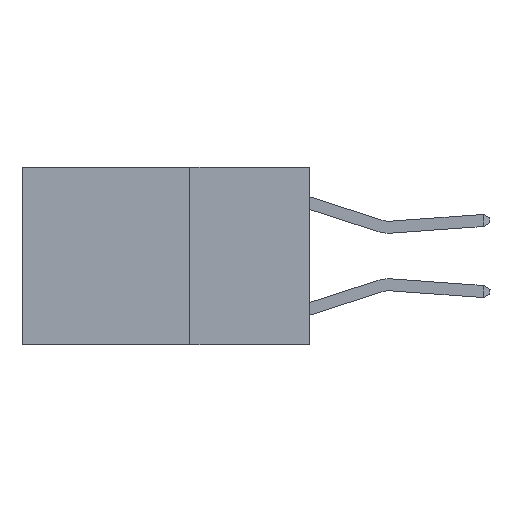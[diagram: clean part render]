
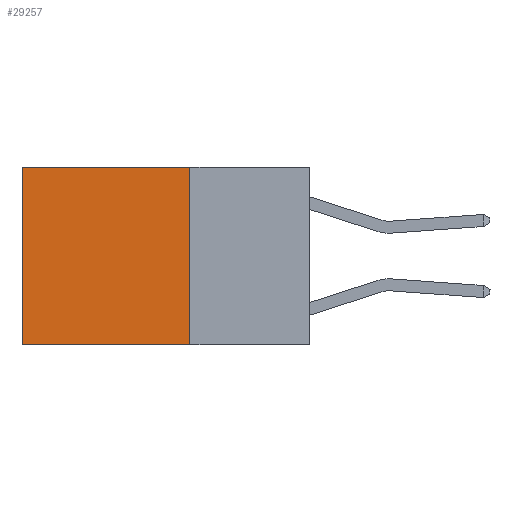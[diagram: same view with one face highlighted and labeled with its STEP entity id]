
A CAD part, left-side view. The second image highlights one B-rep face of the part: STEP entity #29257.
In plain terms, the highlighted planar face has unit normal (-1, 0, 0).
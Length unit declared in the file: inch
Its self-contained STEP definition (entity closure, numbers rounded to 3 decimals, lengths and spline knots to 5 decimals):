
#16 = VERTEX_POINT ( 'NONE', #10404 ) ;
#729 = VECTOR ( 'NONE', #4383, 39.37008 ) ;
#1619 = CARTESIAN_POINT ( 'NONE',  ( 0.2625, 0.25, -0.37 ) ) ;
#1947 = DIRECTION ( 'NONE',  ( 0., 0., -1. ) ) ;
#2571 = AXIS2_PLACEMENT_3D ( 'NONE', #29597, #22573, #27532 ) ;
#2714 = ORIENTED_EDGE ( 'NONE', *, *, #2719, .F. ) ;
#2719 = EDGE_CURVE ( 'NONE', #16, #14542, #9304, .T. ) ;
#4383 = DIRECTION ( 'NONE',  ( 0., 1., 0. ) ) ;
#5448 = FACE_OUTER_BOUND ( 'NONE', #6507, .T. ) ;
#6227 = DIRECTION ( 'NONE',  ( 0., 1., 0. ) ) ;
#6507 = EDGE_LOOP ( 'NONE', ( #23739, #10887, #2714, #9465 ) ) ;
#6659 = VERTEX_POINT ( 'NONE', #13596 ) ;
#7477 = VERTEX_POINT ( 'NONE', #27280 ) ;
#9304 = LINE ( 'NONE', #18592, #24516 ) ;
#9465 = ORIENTED_EDGE ( 'NONE', *, *, #14191, .T. ) ;
#10404 = CARTESIAN_POINT ( 'NONE',  ( 0.2625, 0.25, 0. ) ) ;
#10887 = ORIENTED_EDGE ( 'NONE', *, *, #29329, .F. ) ;
#12687 = LINE ( 'NONE', #27401, #13632 ) ;
#12809 = VECTOR ( 'NONE', #6227, 39.37008 ) ;
#13596 = CARTESIAN_POINT ( 'NONE',  ( 0.2625, 0.6, -0.37 ) ) ;
#13632 = VECTOR ( 'NONE', #22288, 39.37008 ) ;
#14191 = EDGE_CURVE ( 'NONE', #16, #7477, #19114, .T. ) ;
#14542 = VERTEX_POINT ( 'NONE', #27095 ) ;
#18085 = PLANE ( 'NONE',  #2571 ) ;
#18405 = LINE ( 'NONE', #1619, #12809 ) ;
#18592 = CARTESIAN_POINT ( 'NONE',  ( 0.2625, 0.25, 0. ) ) ;
#18810 = CARTESIAN_POINT ( 'NONE',  ( 0.2625, 0.25, 0. ) ) ;
#19114 = LINE ( 'NONE', #18810, #729 ) ;
#22288 = DIRECTION ( 'NONE',  ( 0., 0., -1. ) ) ;
#22573 = DIRECTION ( 'NONE',  ( 1., 0., 0. ) ) ;
#22824 = EDGE_CURVE ( 'NONE', #7477, #6659, #12687, .T. ) ;
#23739 = ORIENTED_EDGE ( 'NONE', *, *, #22824, .T. ) ;
#24516 = VECTOR ( 'NONE', #1947, 39.37008 ) ;
#27095 = CARTESIAN_POINT ( 'NONE',  ( 0.2625, 0.25, -0.37 ) ) ;
#27280 = CARTESIAN_POINT ( 'NONE',  ( 0.2625, 0.6, 0. ) ) ;
#27401 = CARTESIAN_POINT ( 'NONE',  ( 0.2625, 0.6, 0. ) ) ;
#27532 = DIRECTION ( 'NONE',  ( 0., 0., -1. ) ) ;
#29257 = ADVANCED_FACE ( 'NONE', ( #5448 ), #18085, .F. ) ;
#29329 = EDGE_CURVE ( 'NONE', #14542, #6659, #18405, .T. ) ;
#29597 = CARTESIAN_POINT ( 'NONE',  ( 0.2625, 0.25, 0. ) ) ;
